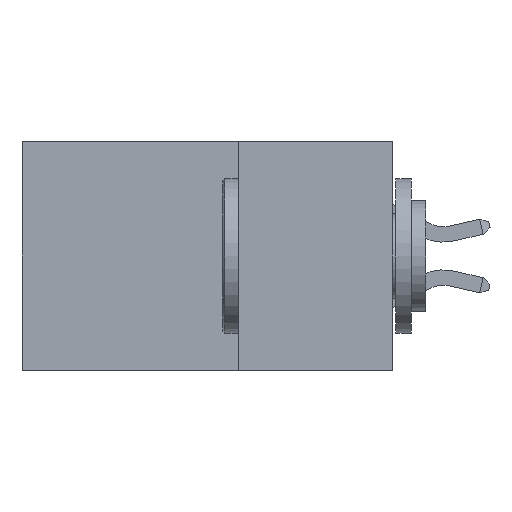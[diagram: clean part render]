
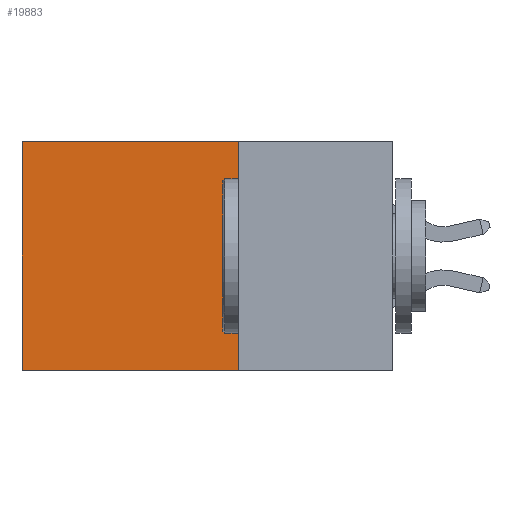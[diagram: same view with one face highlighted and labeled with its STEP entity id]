
A CAD part, left-side view. The second image highlights one B-rep face of the part: STEP entity #19883.
In plain terms, the highlighted planar face has unit normal (-1, 0, 0).
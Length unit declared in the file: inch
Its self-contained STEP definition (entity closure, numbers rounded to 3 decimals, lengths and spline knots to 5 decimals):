
#508 = VECTOR ( 'NONE', #16889, 39.37008 ) ;
#510 = LINE ( 'NONE', #22808, #11359 ) ;
#1146 = EDGE_CURVE ( 'NONE', #23280, #20744, #3106, .T. ) ;
#2604 = ORIENTED_EDGE ( 'NONE', *, *, #23014, .T. ) ;
#3106 = LINE ( 'NONE', #4240, #21432 ) ;
#4160 = ORIENTED_EDGE ( 'NONE', *, *, #1146, .T. ) ;
#4240 = CARTESIAN_POINT ( 'NONE',  ( 0.2875, 0.6, 0. ) ) ;
#4566 = CARTESIAN_POINT ( 'NONE',  ( 0.2875, 0.25, 0. ) ) ;
#4713 = VECTOR ( 'NONE', #13257, 39.37008 ) ;
#6202 = DIRECTION ( 'NONE',  ( 0., 1., 0. ) ) ;
#7073 = VERTEX_POINT ( 'NONE', #10878 ) ;
#8200 = CARTESIAN_POINT ( 'NONE',  ( 0.2875, 0.25, 0. ) ) ;
#8947 = FACE_OUTER_BOUND ( 'NONE', #21127, .T. ) ;
#10878 = CARTESIAN_POINT ( 'NONE',  ( 0.2875, 0.25, 0. ) ) ;
#10910 = DIRECTION ( 'NONE',  ( 0., 0., -1. ) ) ;
#11359 = VECTOR ( 'NONE', #6202, 39.37008 ) ;
#12234 = PLANE ( 'NONE',  #17188 ) ;
#13257 = DIRECTION ( 'NONE',  ( 0., 1., 0. ) ) ;
#14191 = EDGE_CURVE ( 'NONE', #23976, #20744, #510, .T. ) ;
#14716 = CARTESIAN_POINT ( 'NONE',  ( 0.2875, 0.25, 0. ) ) ;
#14739 = DIRECTION ( 'NONE',  ( 0., 0., -1. ) ) ;
#14760 = ORIENTED_EDGE ( 'NONE', *, *, #19097, .F. ) ;
#14897 = LINE ( 'NONE', #4566, #4713 ) ;
#16889 = DIRECTION ( 'NONE',  ( 0., 0., -1. ) ) ;
#17010 = DIRECTION ( 'NONE',  ( 1., 0., 0. ) ) ;
#17188 = AXIS2_PLACEMENT_3D ( 'NONE', #8200, #17010, #14739 ) ;
#18816 = LINE ( 'NONE', #14716, #508 ) ;
#19097 = EDGE_CURVE ( 'NONE', #7073, #23976, #18816, .T. ) ;
#19883 = ADVANCED_FACE ( 'NONE', ( #8947 ), #12234, .F. ) ;
#20744 = VERTEX_POINT ( 'NONE', #24727 ) ;
#21127 = EDGE_LOOP ( 'NONE', ( #4160, #27457, #14760, #2604 ) ) ;
#21432 = VECTOR ( 'NONE', #10910, 39.37008 ) ;
#22189 = CARTESIAN_POINT ( 'NONE',  ( 0.2875, 0.25, -0.37 ) ) ;
#22808 = CARTESIAN_POINT ( 'NONE',  ( 0.2875, 0.25, -0.37 ) ) ;
#23014 = EDGE_CURVE ( 'NONE', #7073, #23280, #14897, .T. ) ;
#23280 = VERTEX_POINT ( 'NONE', #26979 ) ;
#23976 = VERTEX_POINT ( 'NONE', #22189 ) ;
#24727 = CARTESIAN_POINT ( 'NONE',  ( 0.2875, 0.6, -0.37 ) ) ;
#26979 = CARTESIAN_POINT ( 'NONE',  ( 0.2875, 0.6, 0. ) ) ;
#27457 = ORIENTED_EDGE ( 'NONE', *, *, #14191, .F. ) ;
